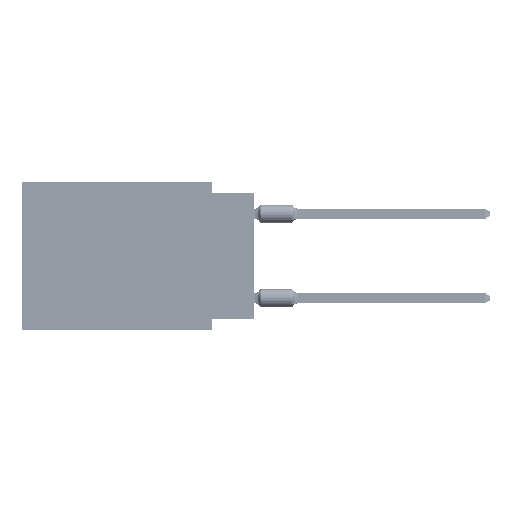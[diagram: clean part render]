
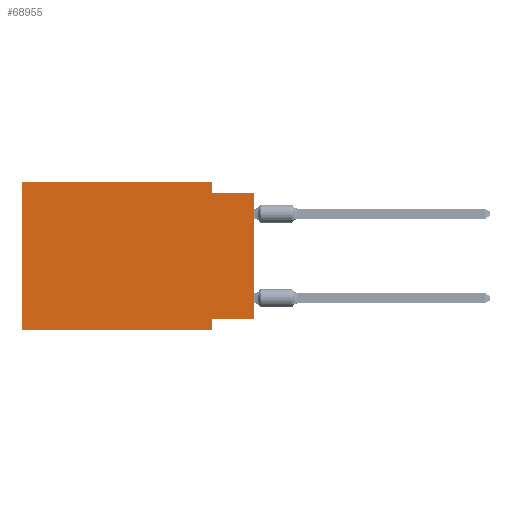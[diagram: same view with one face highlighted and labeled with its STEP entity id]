
A CAD part, left-side view. The second image highlights one B-rep face of the part: STEP entity #68955.
In plain terms, the highlighted planar face has unit normal (-1, 0, 0).
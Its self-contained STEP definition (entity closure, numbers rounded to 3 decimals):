
#1705 = CARTESIAN_POINT ( 'NONE',  ( 0., 13.97, 0. ) ) ;
#1901 = VERTEX_POINT ( 'NONE', #68823 ) ;
#2283 = CARTESIAN_POINT ( 'NONE',  ( 0., 2.54, -0.635 ) ) ;
#4412 = EDGE_CURVE ( 'NONE', #1901, #25167, #95210, .T. ) ;
#5451 = CARTESIAN_POINT ( 'NONE',  ( 0., 0., -8.255 ) ) ;
#9398 = VERTEX_POINT ( 'NONE', #57341 ) ;
#10040 = CARTESIAN_POINT ( 'NONE',  ( 0., 13.97, 0. ) ) ;
#10363 = LINE ( 'NONE', #52397, #53468 ) ;
#11237 = VECTOR ( 'NONE', #51614, 1000. ) ;
#12286 = VECTOR ( 'NONE', #85412, 1000. ) ;
#19243 = EDGE_CURVE ( 'NONE', #74338, #80419, #93134, .T. ) ;
#19448 = DIRECTION ( 'NONE',  ( 0., 0., -1. ) ) ;
#21371 = CARTESIAN_POINT ( 'NONE',  ( 0., 0., -8.255 ) ) ;
#24425 = ORIENTED_EDGE ( 'NONE', *, *, #58397, .T. ) ;
#25167 = VERTEX_POINT ( 'NONE', #78489 ) ;
#25482 = DIRECTION ( 'NONE',  ( 0., 0., 1. ) ) ;
#26683 = CARTESIAN_POINT ( 'NONE',  ( 0., 2.54, 0. ) ) ;
#27760 = PLANE ( 'NONE',  #42184 ) ;
#29077 = DIRECTION ( 'NONE',  ( 0., 0., -1. ) ) ;
#34915 = LINE ( 'NONE', #5451, #71147 ) ;
#35671 = VECTOR ( 'NONE', #90443, 1000. ) ;
#37047 = EDGE_CURVE ( 'NONE', #9398, #74338, #47675, .T. ) ;
#42184 = AXIS2_PLACEMENT_3D ( 'NONE', #72169, #58624, #80344 ) ;
#43121 = CARTESIAN_POINT ( 'NONE',  ( 0., 2.54, 0. ) ) ;
#43185 = FACE_OUTER_BOUND ( 'NONE', #71144, .T. ) ;
#45147 = DIRECTION ( 'NONE',  ( 0., -1., 0. ) ) ;
#45853 = EDGE_CURVE ( 'NONE', #84565, #1901, #34915, .T. ) ;
#47675 = LINE ( 'NONE', #10040, #85415 ) ;
#48523 = VERTEX_POINT ( 'NONE', #68188 ) ;
#49657 = CARTESIAN_POINT ( 'NONE',  ( 0., 13.97, 0. ) ) ;
#50172 = ORIENTED_EDGE ( 'NONE', *, *, #45853, .F. ) ;
#51614 = DIRECTION ( 'NONE',  ( 0., -1., 0. ) ) ;
#52397 = CARTESIAN_POINT ( 'NONE',  ( 0., 0., -0.635 ) ) ;
#53468 = VECTOR ( 'NONE', #45147, 1000. ) ;
#55649 = LINE ( 'NONE', #69655, #35671 ) ;
#57320 = VECTOR ( 'NONE', #19448, 1000. ) ;
#57341 = CARTESIAN_POINT ( 'NONE',  ( 0., 13.97, -8.89 ) ) ;
#58397 = EDGE_CURVE ( 'NONE', #84565, #48523, #55649, .T. ) ;
#58570 = EDGE_CURVE ( 'NONE', #80419, #86894, #64338, .T. ) ;
#58624 = DIRECTION ( 'NONE',  ( 1., 0., 0. ) ) ;
#63819 = ORIENTED_EDGE ( 'NONE', *, *, #4412, .F. ) ;
#64126 = VECTOR ( 'NONE', #29077, 1000. ) ;
#64338 = LINE ( 'NONE', #26683, #57320 ) ;
#64981 = ORIENTED_EDGE ( 'NONE', *, *, #58570, .F. ) ;
#67559 = LINE ( 'NONE', #82498, #11237 ) ;
#68188 = CARTESIAN_POINT ( 'NONE',  ( 0., 0., -0.635 ) ) ;
#68823 = CARTESIAN_POINT ( 'NONE',  ( 0., 2.54, -8.255 ) ) ;
#68955 = ADVANCED_FACE ( 'NONE', ( #43185 ), #27760, .F. ) ;
#69655 = CARTESIAN_POINT ( 'NONE',  ( 0., 0., 0. ) ) ;
#69964 = EDGE_CURVE ( 'NONE', #9398, #25167, #67559, .T. ) ;
#71144 = EDGE_LOOP ( 'NONE', ( #24425, #76185, #64981, #81179, #71901, #72858, #63819, #50172 ) ) ;
#71147 = VECTOR ( 'NONE', #80232, 1000. ) ;
#71901 = ORIENTED_EDGE ( 'NONE', *, *, #37047, .F. ) ;
#72169 = CARTESIAN_POINT ( 'NONE',  ( 0., 13.97, 0. ) ) ;
#72858 = ORIENTED_EDGE ( 'NONE', *, *, #69964, .T. ) ;
#74209 = EDGE_CURVE ( 'NONE', #86894, #48523, #10363, .T. ) ;
#74338 = VERTEX_POINT ( 'NONE', #1705 ) ;
#76185 = ORIENTED_EDGE ( 'NONE', *, *, #74209, .F. ) ;
#78489 = CARTESIAN_POINT ( 'NONE',  ( 0., 2.54, -8.89 ) ) ;
#80232 = DIRECTION ( 'NONE',  ( 0., 1., 0. ) ) ;
#80344 = DIRECTION ( 'NONE',  ( 0., 0., -1. ) ) ;
#80419 = VERTEX_POINT ( 'NONE', #43121 ) ;
#81179 = ORIENTED_EDGE ( 'NONE', *, *, #19243, .F. ) ;
#82498 = CARTESIAN_POINT ( 'NONE',  ( 0., 13.97, -8.89 ) ) ;
#84565 = VERTEX_POINT ( 'NONE', #21371 ) ;
#85412 = DIRECTION ( 'NONE',  ( 0., -1., 0. ) ) ;
#85415 = VECTOR ( 'NONE', #25482, 1000. ) ;
#86894 = VERTEX_POINT ( 'NONE', #2283 ) ;
#87964 = CARTESIAN_POINT ( 'NONE',  ( 0., 2.54, -8.89 ) ) ;
#90443 = DIRECTION ( 'NONE',  ( 0., 0., 1. ) ) ;
#93134 = LINE ( 'NONE', #49657, #12286 ) ;
#95210 = LINE ( 'NONE', #87964, #64126 ) ;
